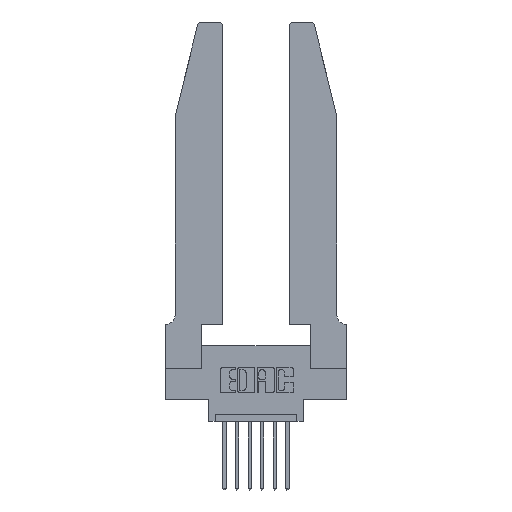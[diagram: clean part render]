
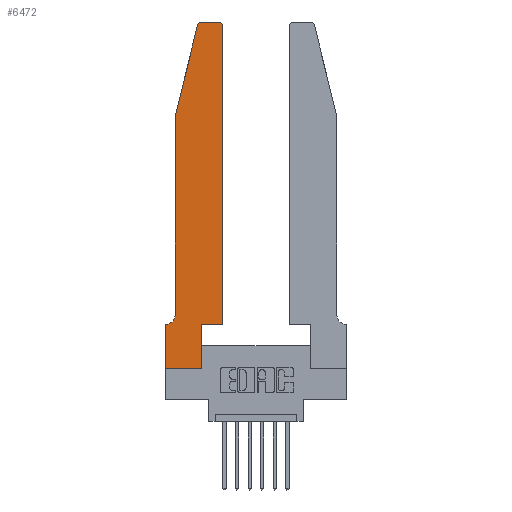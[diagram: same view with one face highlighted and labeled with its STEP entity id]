
A CAD part, top view. The second image highlights one B-rep face of the part: STEP entity #6472.
In plain terms, the highlighted planar face has unit normal (0, 0, 1).
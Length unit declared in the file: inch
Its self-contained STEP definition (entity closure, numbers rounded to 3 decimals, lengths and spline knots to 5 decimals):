
#36 = LINE ( 'NONE', #12227, #5533 ) ;
#97 = EDGE_CURVE ( 'NONE', #1872, #894, #14016, .T. ) ;
#108 = VERTEX_POINT ( 'NONE', #6378 ) ;
#290 = LINE ( 'NONE', #10998, #1815 ) ;
#379 = VECTOR ( 'NONE', #10167, 39.37008 ) ;
#521 = ORIENTED_EDGE ( 'NONE', *, *, #5020, .T. ) ;
#894 = VERTEX_POINT ( 'NONE', #2554 ) ;
#1027 = LINE ( 'NONE', #5128, #9150 ) ;
#1244 = CARTESIAN_POINT ( 'NONE',  ( 0.2605, 2.75, 0.37 ) ) ;
#1342 = VERTEX_POINT ( 'NONE', #6249 ) ;
#1487 = CARTESIAN_POINT ( 'NONE',  ( 0.25487, 2.72718, 0.37 ) ) ;
#1815 = VECTOR ( 'NONE', #10954, 39.37008 ) ;
#1872 = VERTEX_POINT ( 'NONE', #1487 ) ;
#1892 = CARTESIAN_POINT ( 'NONE',  ( 0.4205, 2.72, 0.37 ) ) ;
#1947 = EDGE_CURVE ( 'NONE', #894, #13105, #36, .T. ) ;
#2051 = LINE ( 'NONE', #7672, #10186 ) ;
#2330 = CARTESIAN_POINT ( 'NONE',  ( 0.4205, 2.75, 0.37 ) ) ;
#2427 = EDGE_CURVE ( 'NONE', #3816, #1872, #4331, .T. ) ;
#2554 = CARTESIAN_POINT ( 'NONE',  ( 0.0755, 2., 0.37 ) ) ;
#2685 = FACE_OUTER_BOUND ( 'NONE', #3423, .T. ) ;
#2864 = VERTEX_POINT ( 'NONE', #6529 ) ;
#3080 = DIRECTION ( 'NONE',  ( -0.239, -0.971, 0. ) ) ;
#3241 = DIRECTION ( 'NONE',  ( 1., 0., 0. ) ) ;
#3269 = ORIENTED_EDGE ( 'NONE', *, *, #12949, .T. ) ;
#3377 = EDGE_CURVE ( 'NONE', #12588, #2864, #13511, .T. ) ;
#3418 = DIRECTION ( 'NONE',  ( 0., 0., 1. ) ) ;
#3423 = EDGE_LOOP ( 'NONE', ( #3269, #7590, #7459, #3671, #6999, #4159, #9740, #11808, #12119, #14112, #6834, #521 ) ) ;
#3431 = CARTESIAN_POINT ( 'NONE',  ( 0., 0., 0.37 ) ) ;
#3671 = ORIENTED_EDGE ( 'NONE', *, *, #1947, .T. ) ;
#3816 = VERTEX_POINT ( 'NONE', #4826 ) ;
#3890 = DIRECTION ( 'NONE',  ( 1., 0., 0. ) ) ;
#3964 = DIRECTION ( 'NONE',  ( 0., 0., -1. ) ) ;
#4024 = LINE ( 'NONE', #7913, #5792 ) ;
#4029 = VERTEX_POINT ( 'NONE', #10664 ) ;
#4056 = LINE ( 'NONE', #8065, #5113 ) ;
#4159 = ORIENTED_EDGE ( 'NONE', *, *, #4729, .T. ) ;
#4308 = VECTOR ( 'NONE', #3080, 39.37008 ) ;
#4331 = CIRCLE ( 'NONE', #8457, 0.03 ) ;
#4418 = EDGE_CURVE ( 'NONE', #108, #1342, #2051, .T. ) ;
#4715 = EDGE_CURVE ( 'NONE', #13105, #11953, #5701, .T. ) ;
#4729 = EDGE_CURVE ( 'NONE', #11953, #9238, #1027, .T. ) ;
#4826 = CARTESIAN_POINT ( 'NONE',  ( 0.284, 2.75, 0.37 ) ) ;
#5020 = EDGE_CURVE ( 'NONE', #1342, #6428, #11211, .T. ) ;
#5113 = VECTOR ( 'NONE', #12273, 39.37008 ) ;
#5128 = CARTESIAN_POINT ( 'NONE',  ( 0.0755, 0.35, 0.37 ) ) ;
#5181 = DIRECTION ( 'NONE',  ( -1., 0., 0. ) ) ;
#5533 = VECTOR ( 'NONE', #7813, 39.37008 ) ;
#5701 = CIRCLE ( 'NONE', #10520, 0.07 ) ;
#5792 = VECTOR ( 'NONE', #6695, 39.37008 ) ;
#5816 = EDGE_CURVE ( 'NONE', #4029, #108, #4056, .T. ) ;
#6249 = CARTESIAN_POINT ( 'NONE',  ( 0.4505, 2.72, 0.37 ) ) ;
#6378 = CARTESIAN_POINT ( 'NONE',  ( 0.4505, 0.35, 0.37 ) ) ;
#6428 = VERTEX_POINT ( 'NONE', #2330 ) ;
#6472 = ADVANCED_FACE ( 'NONE', ( #2685 ), #6571, .T. ) ;
#6529 = CARTESIAN_POINT ( 'NONE',  ( 0.2865, 0., 0.37 ) ) ;
#6571 = PLANE ( 'NONE',  #14236 ) ;
#6650 = DIRECTION ( 'NONE',  ( 0., 0., 1. ) ) ;
#6695 = DIRECTION ( 'NONE',  ( 0., -1., 0. ) ) ;
#6834 = ORIENTED_EDGE ( 'NONE', *, *, #4418, .T. ) ;
#6999 = ORIENTED_EDGE ( 'NONE', *, *, #4715, .T. ) ;
#7027 = EDGE_CURVE ( 'NONE', #9238, #12588, #4024, .T. ) ;
#7459 = ORIENTED_EDGE ( 'NONE', *, *, #97, .T. ) ;
#7477 = DIRECTION ( 'NONE',  ( 0., 1., 0. ) ) ;
#7573 = EDGE_CURVE ( 'NONE', #2864, #4029, #290, .T. ) ;
#7590 = ORIENTED_EDGE ( 'NONE', *, *, #2427, .T. ) ;
#7639 = DIRECTION ( 'NONE',  ( 1., 0., 0. ) ) ;
#7672 = CARTESIAN_POINT ( 'NONE',  ( 0.4505, 0.35, 0.37 ) ) ;
#7813 = DIRECTION ( 'NONE',  ( 0., -1., 0. ) ) ;
#7913 = CARTESIAN_POINT ( 'NONE',  ( 0., 0., 0.37 ) ) ;
#7984 = CARTESIAN_POINT ( 'NONE',  ( 0.0055, 0.35, 0.37 ) ) ;
#8065 = CARTESIAN_POINT ( 'NONE',  ( 0.4505, 0.35, 0.37 ) ) ;
#8457 = AXIS2_PLACEMENT_3D ( 'NONE', #13294, #6650, #3241 ) ;
#8630 = VECTOR ( 'NONE', #10191, 39.37008 ) ;
#8789 = CARTESIAN_POINT ( 'NONE',  ( 0., 0.35, 0.37 ) ) ;
#9016 = CARTESIAN_POINT ( 'NONE',  ( 0., 0.35, 0.37 ) ) ;
#9076 = CARTESIAN_POINT ( 'NONE',  ( 0., 0., 0.37 ) ) ;
#9150 = VECTOR ( 'NONE', #5181, 39.37008 ) ;
#9238 = VERTEX_POINT ( 'NONE', #9016 ) ;
#9740 = ORIENTED_EDGE ( 'NONE', *, *, #7027, .T. ) ;
#10167 = DIRECTION ( 'NONE',  ( 1., 0., 0. ) ) ;
#10186 = VECTOR ( 'NONE', #7477, 39.37008 ) ;
#10191 = DIRECTION ( 'NONE',  ( -1., 0., 0. ) ) ;
#10520 = AXIS2_PLACEMENT_3D ( 'NONE', #10613, #3964, #11772 ) ;
#10613 = CARTESIAN_POINT ( 'NONE',  ( 0.0055, 0.42, 0.37 ) ) ;
#10664 = CARTESIAN_POINT ( 'NONE',  ( 0.2865, 0.35, 0.37 ) ) ;
#10674 = DIRECTION ( 'NONE',  ( 0., 0., 1. ) ) ;
#10954 = DIRECTION ( 'NONE',  ( 0., 1., 0. ) ) ;
#10998 = CARTESIAN_POINT ( 'NONE',  ( 0.2865, 0.35, 0.37 ) ) ;
#11211 = CIRCLE ( 'NONE', #12711, 0.03 ) ;
#11582 = LINE ( 'NONE', #1244, #8630 ) ;
#11772 = DIRECTION ( 'NONE',  ( -1., 0., 0. ) ) ;
#11808 = ORIENTED_EDGE ( 'NONE', *, *, #3377, .T. ) ;
#11953 = VERTEX_POINT ( 'NONE', #7984 ) ;
#12119 = ORIENTED_EDGE ( 'NONE', *, *, #7573, .T. ) ;
#12227 = CARTESIAN_POINT ( 'NONE',  ( 0.0755, 2., 0.37 ) ) ;
#12273 = DIRECTION ( 'NONE',  ( 1., 0., 0. ) ) ;
#12588 = VERTEX_POINT ( 'NONE', #9076 ) ;
#12600 = CARTESIAN_POINT ( 'NONE',  ( 0.0755, 0.42, 0.37 ) ) ;
#12711 = AXIS2_PLACEMENT_3D ( 'NONE', #1892, #10674, #3890 ) ;
#12949 = EDGE_CURVE ( 'NONE', #6428, #3816, #11582, .T. ) ;
#12995 = CARTESIAN_POINT ( 'NONE',  ( 0.0755, 2., 0.37 ) ) ;
#13105 = VERTEX_POINT ( 'NONE', #12600 ) ;
#13294 = CARTESIAN_POINT ( 'NONE',  ( 0.284, 2.72, 0.37 ) ) ;
#13511 = LINE ( 'NONE', #3431, #379 ) ;
#14016 = LINE ( 'NONE', #12995, #4308 ) ;
#14112 = ORIENTED_EDGE ( 'NONE', *, *, #5816, .T. ) ;
#14236 = AXIS2_PLACEMENT_3D ( 'NONE', #8789, #3418, #7639 ) ;
